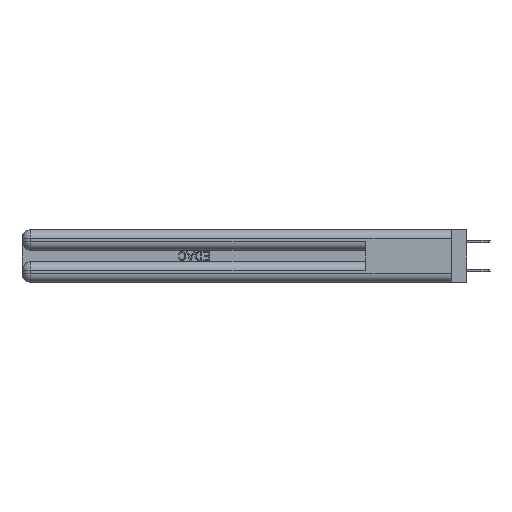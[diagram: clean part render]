
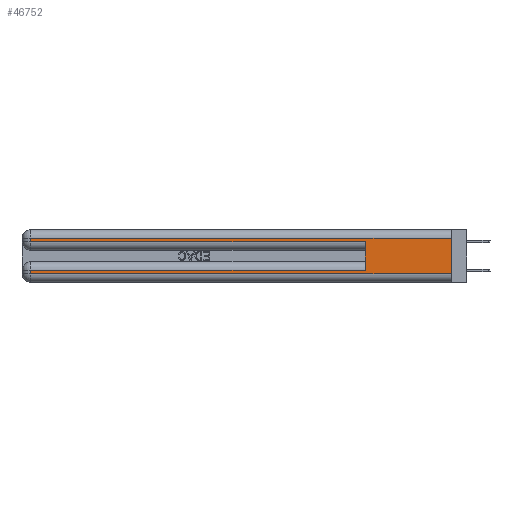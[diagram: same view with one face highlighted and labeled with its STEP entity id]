
A CAD part, left-side view. The second image highlights one B-rep face of the part: STEP entity #46752.
In plain terms, the highlighted planar face has unit normal (-1, 0, 0).
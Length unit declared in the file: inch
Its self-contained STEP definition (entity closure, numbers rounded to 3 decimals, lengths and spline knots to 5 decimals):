
#218 = FACE_OUTER_BOUND ( 'NONE', #48932, .T. ) ;
#2977 = ORIENTED_EDGE ( 'NONE', *, *, #10016, .F. ) ;
#3333 = VECTOR ( 'NONE', #16810, 39.37008 ) ;
#4478 = CARTESIAN_POINT ( 'NONE',  ( 0., 0., 0.31 ) ) ;
#4558 = LINE ( 'NONE', #47560, #3333 ) ;
#5338 = CARTESIAN_POINT ( 'NONE',  ( 0., 2.94, 0.37 ) ) ;
#6549 = CARTESIAN_POINT ( 'NONE',  ( 0., 0., 0.37 ) ) ;
#7801 = LINE ( 'NONE', #16228, #27223 ) ;
#8804 = CARTESIAN_POINT ( 'NONE',  ( 0., 0., 0.085 ) ) ;
#9681 = EDGE_CURVE ( 'NONE', #36814, #40634, #13366, .T. ) ;
#10016 = EDGE_CURVE ( 'NONE', #31304, #48958, #7801, .T. ) ;
#10496 = DIRECTION ( 'NONE',  ( 0., 0., -1. ) ) ;
#10634 = CARTESIAN_POINT ( 'NONE',  ( 0., 0.6, 0.085 ) ) ;
#12007 = VECTOR ( 'NONE', #12752, 39.37008 ) ;
#12011 = LINE ( 'NONE', #13536, #31350 ) ;
#12137 = VECTOR ( 'NONE', #25168, 39.37008 ) ;
#12752 = DIRECTION ( 'NONE',  ( 0., 1., 0. ) ) ;
#12840 = CARTESIAN_POINT ( 'NONE',  ( 0., 0., 0.285 ) ) ;
#13366 = LINE ( 'NONE', #44362, #12137 ) ;
#13536 = CARTESIAN_POINT ( 'NONE',  ( 0., 0., 0.37 ) ) ;
#13876 = EDGE_CURVE ( 'NONE', #33470, #40441, #33435, .T. ) ;
#15920 = VECTOR ( 'NONE', #25795, 39.37008 ) ;
#16228 = CARTESIAN_POINT ( 'NONE',  ( 0., 0.6, 0.145 ) ) ;
#16249 = EDGE_CURVE ( 'NONE', #40441, #25251, #4558, .T. ) ;
#16810 = DIRECTION ( 'NONE',  ( 0., -1., 0. ) ) ;
#17436 = DIRECTION ( 'NONE',  ( 0., 0., -1. ) ) ;
#18049 = CARTESIAN_POINT ( 'NONE',  ( 0., 0., 0.31 ) ) ;
#23162 = VECTOR ( 'NONE', #40260, 39.37008 ) ;
#23242 = ORIENTED_EDGE ( 'NONE', *, *, #28437, .T. ) ;
#23720 = ORIENTED_EDGE ( 'NONE', *, *, #13876, .T. ) ;
#23940 = DIRECTION ( 'NONE',  ( 0., 0., 1. ) ) ;
#24725 = EDGE_CURVE ( 'NONE', #25895, #25251, #12011, .T. ) ;
#24812 = CARTESIAN_POINT ( 'NONE',  ( 0., 2.94, 0.085 ) ) ;
#25168 = DIRECTION ( 'NONE',  ( 0., 0., -1. ) ) ;
#25251 = VERTEX_POINT ( 'NONE', #43318 ) ;
#25358 = ORIENTED_EDGE ( 'NONE', *, *, #34759, .T. ) ;
#25795 = DIRECTION ( 'NONE',  ( 0., 1., 0. ) ) ;
#25895 = VERTEX_POINT ( 'NONE', #4478 ) ;
#26052 = ORIENTED_EDGE ( 'NONE', *, *, #9681, .T. ) ;
#27223 = VECTOR ( 'NONE', #23940, 39.37008 ) ;
#27937 = AXIS2_PLACEMENT_3D ( 'NONE', #6549, #33649, #10496 ) ;
#28309 = CARTESIAN_POINT ( 'NONE',  ( 0., 2.94, 0.285 ) ) ;
#28437 = EDGE_CURVE ( 'NONE', #40634, #48958, #42953, .T. ) ;
#29817 = PLANE ( 'NONE',  #27937 ) ;
#31304 = VERTEX_POINT ( 'NONE', #10634 ) ;
#31350 = VECTOR ( 'NONE', #17436, 39.37008 ) ;
#31515 = VECTOR ( 'NONE', #43666, 39.37008 ) ;
#33435 = LINE ( 'NONE', #5338, #23162 ) ;
#33470 = VERTEX_POINT ( 'NONE', #24812 ) ;
#33649 = DIRECTION ( 'NONE',  ( 1., 0., 0. ) ) ;
#34759 = EDGE_CURVE ( 'NONE', #31304, #33470, #42774, .T. ) ;
#34862 = CARTESIAN_POINT ( 'NONE',  ( 0., 2.94, 0.06 ) ) ;
#35376 = ORIENTED_EDGE ( 'NONE', *, *, #46077, .T. ) ;
#36112 = ORIENTED_EDGE ( 'NONE', *, *, #24725, .F. ) ;
#36439 = LINE ( 'NONE', #18049, #15920 ) ;
#36814 = VERTEX_POINT ( 'NONE', #46383 ) ;
#40260 = DIRECTION ( 'NONE',  ( 0., 0., -1. ) ) ;
#40441 = VERTEX_POINT ( 'NONE', #34862 ) ;
#40634 = VERTEX_POINT ( 'NONE', #28309 ) ;
#41573 = ORIENTED_EDGE ( 'NONE', *, *, #16249, .T. ) ;
#42774 = LINE ( 'NONE', #8804, #12007 ) ;
#42953 = LINE ( 'NONE', #12840, #31515 ) ;
#43318 = CARTESIAN_POINT ( 'NONE',  ( 0., 0., 0.06 ) ) ;
#43666 = DIRECTION ( 'NONE',  ( 0., -1., 0. ) ) ;
#44362 = CARTESIAN_POINT ( 'NONE',  ( 0., 2.94, 0.37 ) ) ;
#46077 = EDGE_CURVE ( 'NONE', #25895, #36814, #36439, .T. ) ;
#46383 = CARTESIAN_POINT ( 'NONE',  ( 0., 2.94, 0.31 ) ) ;
#46752 = ADVANCED_FACE ( 'NONE', ( #218 ), #29817, .F. ) ;
#47560 = CARTESIAN_POINT ( 'NONE',  ( 0., 0., 0.06 ) ) ;
#48932 = EDGE_LOOP ( 'NONE', ( #36112, #35376, #26052, #23242, #2977, #25358, #23720, #41573 ) ) ;
#48958 = VERTEX_POINT ( 'NONE', #49292 ) ;
#49292 = CARTESIAN_POINT ( 'NONE',  ( 0., 0.6, 0.285 ) ) ;
